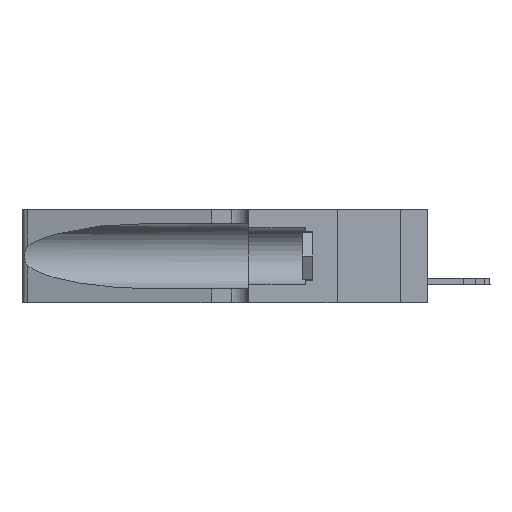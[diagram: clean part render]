
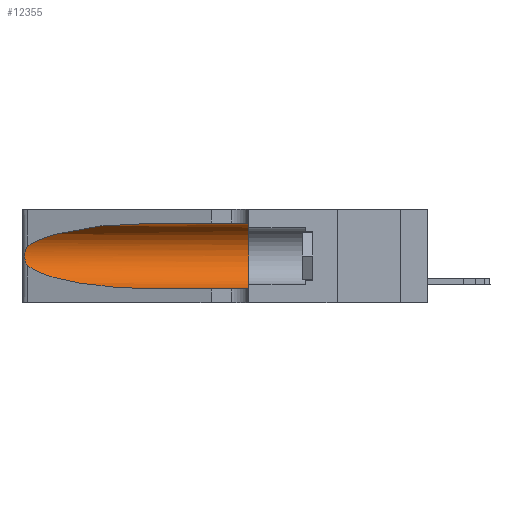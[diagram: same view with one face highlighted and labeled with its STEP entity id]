
A CAD part, left-side view. The second image highlights one B-rep face of the part: STEP entity #12355.
In plain terms, the highlighted cylindrical face has radius 3.308 mm (diameter 6.617 mm), a partial arc.
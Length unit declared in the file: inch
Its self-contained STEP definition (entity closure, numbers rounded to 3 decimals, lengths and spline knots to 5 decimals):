
#126 = CIRCLE ( 'NONE', #10302, 0.13025 ) ;
#148 = VECTOR ( 'NONE', #12668, 39.37008 ) ;
#290 = CARTESIAN_POINT ( 'NONE',  ( 0.1305, 1.61858, 0.31525 ) ) ;
#641 = CARTESIAN_POINT ( 'NONE',  ( 0.25787, 1.23484, 0.2124 ) ) ;
#1224 = AXIS2_PLACEMENT_3D ( 'NONE', #19107, #6742, #12875 ) ;
#1532 = DIRECTION ( 'NONE',  ( 0., 1., 0. ) ) ;
#2197 = CARTESIAN_POINT ( 'NONE',  ( 0.25639, 1.23184, 0.21858 ) ) ;
#2271 = CARTESIAN_POINT ( 'NONE',  ( 0.25487, 1.22718, 0.14631 ) ) ;
#2305 = CARTESIAN_POINT ( 'NONE',  ( 0.1305, 0.35, 0.31525 ) ) ;
#2343 = LINE ( 'NONE', #290, #148 ) ;
#2472 = CARTESIAN_POINT ( 'NONE',  ( 0.25854, 1.2359, 0.20912 ) ) ;
#2537 = CARTESIAN_POINT ( 'NONE',  ( 0.18966, 0.96281, 0.31525 ) ) ;
#2568 = EDGE_CURVE ( 'NONE', #16431, #9391, #15080, .T. ) ;
#2580 = DIRECTION ( 'NONE',  ( 0., -1., 0. ) ) ;
#3214 = VECTOR ( 'NONE', #2580, 39.37008 ) ;
#3586 = CYLINDRICAL_SURFACE ( 'NONE', #1224, 0.13025 ) ;
#4051 = CARTESIAN_POINT ( 'NONE',  ( 0.26018, 1.23835, 0.19895 ) ) ;
#4385 = EDGE_CURVE ( 'NONE', #8562, #11256, #5958, .T. ) ;
#4601 = CARTESIAN_POINT ( 'NONE',  ( 0.1305, 0.72297, 0.31525 ) ) ;
#5006 = EDGE_CURVE ( 'NONE', #9391, #8562, #7229, .T. ) ;
#5359 = CARTESIAN_POINT ( 'NONE',  ( 0.25555, 1.22993, 0.14849 ) ) ;
#5532 = ORIENTED_EDGE ( 'NONE', *, *, #9698, .T. ) ;
#5626 = CARTESIAN_POINT ( 'NONE',  ( 0.25856, 1.23593, 0.16098 ) ) ;
#5675 = CARTESIAN_POINT ( 'NONE',  ( 0.25487, 1.22718, 0.22369 ) ) ;
#5958 =( BOUNDED_CURVE ( )  B_SPLINE_CURVE ( 3, ( #11421, #17752, #8481, #6698 ),
 .UNSPECIFIED., .F., .T. ) 
 B_SPLINE_CURVE_WITH_KNOTS ( ( 4, 4 ),
 ( 3.44316, 4.71239 ),
 .UNSPECIFIED. ) 
 CURVE ( )  GEOMETRIC_REPRESENTATION_ITEM ( )  RATIONAL_B_SPLINE_CURVE ( ( 1., 0.87, 0.87, 1. ) ) 
 REPRESENTATION_ITEM ( '' )  );
#5975 = CARTESIAN_POINT ( 'NONE',  ( 0.2373, 1.15595, 0.28018 ) ) ;
#6698 = CARTESIAN_POINT ( 'NONE',  ( 0.1305, 0.72297, 0.05475 ) ) ;
#6742 = DIRECTION ( 'NONE',  ( 0., -1., 0. ) ) ;
#7032 = CARTESIAN_POINT ( 'NONE',  ( 0.25789, 1.23486, 0.15765 ) ) ;
#7229 = B_SPLINE_CURVE_WITH_KNOTS ( 'NONE', 3,
 ( #14839, #16530, #2197, #641, #2472, #4051, #14911, #18011, #16397, #5626, #7032, #17941, #5359, #2271 ),
 .UNSPECIFIED., .F., .F.,
 ( 4, 2, 2, 2, 2, 2, 4 ),
 ( 0., 0.00027, 0.00053, 0.00107, 0.0016, 0.00187, 0.00214 ),
 .UNSPECIFIED. ) ;
#7376 = ORIENTED_EDGE ( 'NONE', *, *, #18812, .F. ) ;
#7410 = LINE ( 'NONE', #19711, #3214 ) ;
#7557 = CARTESIAN_POINT ( 'NONE',  ( 0.25487, 1.22718, 0.22369 ) ) ;
#7650 = CARTESIAN_POINT ( 'NONE',  ( 0.1305, 0.35, 0.185 ) ) ;
#7926 = ORIENTED_EDGE ( 'NONE', *, *, #12427, .F. ) ;
#8481 = CARTESIAN_POINT ( 'NONE',  ( 0.18966, 0.96281, 0.05475 ) ) ;
#8562 = VERTEX_POINT ( 'NONE', #11685 ) ;
#8714 = CARTESIAN_POINT ( 'NONE',  ( 0.1305, 0.35, 0.05475 ) ) ;
#9391 = VERTEX_POINT ( 'NONE', #5675 ) ;
#9698 = EDGE_CURVE ( 'NONE', #11256, #10109, #7410, .T. ) ;
#10109 = VERTEX_POINT ( 'NONE', #8714 ) ;
#10302 = AXIS2_PLACEMENT_3D ( 'NONE', #7650, #1532, #20044 ) ;
#11256 = VERTEX_POINT ( 'NONE', #18715 ) ;
#11421 = CARTESIAN_POINT ( 'NONE',  ( 0.25487, 1.22718, 0.14631 ) ) ;
#11685 = CARTESIAN_POINT ( 'NONE',  ( 0.25487, 1.22718, 0.14631 ) ) ;
#12355 = ADVANCED_FACE ( 'NONE', ( #15063 ), #3586, .F. ) ;
#12427 = EDGE_CURVE ( 'NONE', #16431, #17604, #2343, .T. ) ;
#12668 = DIRECTION ( 'NONE',  ( 0., -1., 0. ) ) ;
#12875 = DIRECTION ( 'NONE',  ( 0., 0., -1. ) ) ;
#13444 = ORIENTED_EDGE ( 'NONE', *, *, #5006, .T. ) ;
#14059 = ORIENTED_EDGE ( 'NONE', *, *, #2568, .T. ) ;
#14839 = CARTESIAN_POINT ( 'NONE',  ( 0.25487, 1.22718, 0.22369 ) ) ;
#14911 = CARTESIAN_POINT ( 'NONE',  ( 0.26075, 1.23896, 0.19203 ) ) ;
#15063 = FACE_OUTER_BOUND ( 'NONE', #19319, .T. ) ;
#15080 =( BOUNDED_CURVE ( )  B_SPLINE_CURVE ( 3, ( #15110, #2537, #5975, #7557 ),
 .UNSPECIFIED., .F., .T. ) 
 B_SPLINE_CURVE_WITH_KNOTS ( ( 4, 4 ),
 ( 1.5708, 2.84003 ),
 .UNSPECIFIED. ) 
 CURVE ( )  GEOMETRIC_REPRESENTATION_ITEM ( )  RATIONAL_B_SPLINE_CURVE ( ( 1., 0.87, 0.87, 1. ) ) 
 REPRESENTATION_ITEM ( '' )  );
#15110 = CARTESIAN_POINT ( 'NONE',  ( 0.1305, 0.72297, 0.31525 ) ) ;
#16397 = CARTESIAN_POINT ( 'NONE',  ( 0.26017, 1.23833, 0.17102 ) ) ;
#16431 = VERTEX_POINT ( 'NONE', #4601 ) ;
#16530 = CARTESIAN_POINT ( 'NONE',  ( 0.25555, 1.22994, 0.2215 ) ) ;
#17604 = VERTEX_POINT ( 'NONE', #2305 ) ;
#17752 = CARTESIAN_POINT ( 'NONE',  ( 0.2373, 1.15595, 0.08982 ) ) ;
#17941 = CARTESIAN_POINT ( 'NONE',  ( 0.25639, 1.23186, 0.15144 ) ) ;
#18011 = CARTESIAN_POINT ( 'NONE',  ( 0.26075, 1.23896, 0.178 ) ) ;
#18715 = CARTESIAN_POINT ( 'NONE',  ( 0.1305, 0.72297, 0.05475 ) ) ;
#18812 = EDGE_CURVE ( 'NONE', #17604, #10109, #126, .T. ) ;
#19107 = CARTESIAN_POINT ( 'NONE',  ( 0.1305, 1.61858, 0.185 ) ) ;
#19319 = EDGE_LOOP ( 'NONE', ( #14059, #13444, #19404, #5532, #7376, #7926 ) ) ;
#19404 = ORIENTED_EDGE ( 'NONE', *, *, #4385, .T. ) ;
#19711 = CARTESIAN_POINT ( 'NONE',  ( 0.1305, 1.61858, 0.05475 ) ) ;
#20044 = DIRECTION ( 'NONE',  ( 0., 0., 1. ) ) ;
